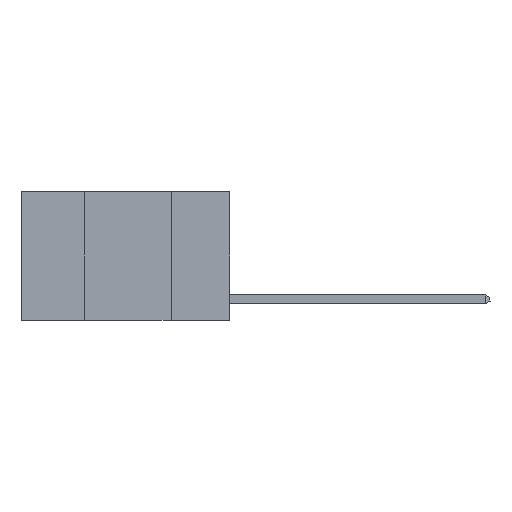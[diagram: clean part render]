
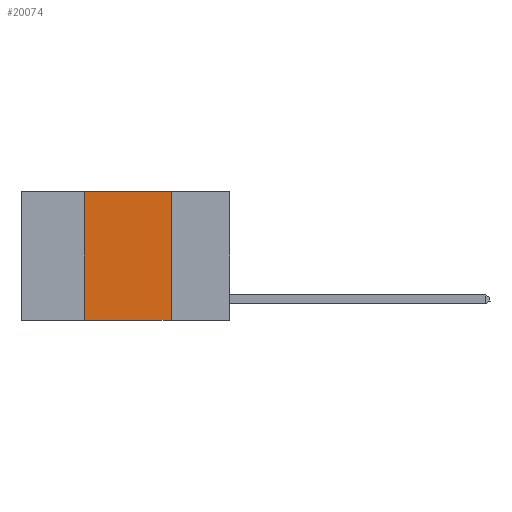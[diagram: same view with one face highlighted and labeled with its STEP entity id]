
A CAD part, left-side view. The second image highlights one B-rep face of the part: STEP entity #20074.
In plain terms, the highlighted planar face has unit normal (-1, 0, 0).
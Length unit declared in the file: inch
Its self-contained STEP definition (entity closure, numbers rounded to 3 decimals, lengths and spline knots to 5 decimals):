
#1124 = ORIENTED_EDGE ( 'NONE', *, *, #6779, .F. ) ;
#2947 = VERTEX_POINT ( 'NONE', #5891 ) ;
#3557 = ORIENTED_EDGE ( 'NONE', *, *, #16821, .T. ) ;
#3679 = VERTEX_POINT ( 'NONE', #15670 ) ;
#3696 = CARTESIAN_POINT ( 'NONE',  ( 0., 0.6, 0. ) ) ;
#5827 = VECTOR ( 'NONE', #14169, 39.37008 ) ;
#5891 = CARTESIAN_POINT ( 'NONE',  ( 0., 0.17, -0.37 ) ) ;
#6779 = EDGE_CURVE ( 'NONE', #3679, #17663, #15502, .T. ) ;
#7048 = CARTESIAN_POINT ( 'NONE',  ( 0., 0.6, 0. ) ) ;
#7406 = AXIS2_PLACEMENT_3D ( 'NONE', #7048, #8895, #21482 ) ;
#7772 = VECTOR ( 'NONE', #23227, 39.37008 ) ;
#7928 = VERTEX_POINT ( 'NONE', #10152 ) ;
#8895 = DIRECTION ( 'NONE',  ( 1., 0., 0. ) ) ;
#9037 = LINE ( 'NONE', #9591, #18083 ) ;
#9591 = CARTESIAN_POINT ( 'NONE',  ( 0., 0.17, 0. ) ) ;
#9761 = CARTESIAN_POINT ( 'NONE',  ( 0., 0.42, 0. ) ) ;
#10152 = CARTESIAN_POINT ( 'NONE',  ( 0., 0.17, 0. ) ) ;
#10244 = EDGE_CURVE ( 'NONE', #17663, #7928, #10326, .T. ) ;
#10326 = LINE ( 'NONE', #3696, #19339 ) ;
#12634 = LINE ( 'NONE', #16142, #7772 ) ;
#14169 = DIRECTION ( 'NONE',  ( 0., 0., 1. ) ) ;
#14608 = DIRECTION ( 'NONE',  ( 0., -1., 0. ) ) ;
#14782 = EDGE_CURVE ( 'NONE', #7928, #2947, #9037, .T. ) ;
#15502 = LINE ( 'NONE', #15904, #5827 ) ;
#15670 = CARTESIAN_POINT ( 'NONE',  ( 0., 0.42, -0.37 ) ) ;
#15904 = CARTESIAN_POINT ( 'NONE',  ( 0., 0.42, 0. ) ) ;
#16142 = CARTESIAN_POINT ( 'NONE',  ( 0., 0.6, -0.37 ) ) ;
#16821 = EDGE_CURVE ( 'NONE', #3679, #2947, #12634, .T. ) ;
#17663 = VERTEX_POINT ( 'NONE', #9761 ) ;
#17904 = PLANE ( 'NONE',  #7406 ) ;
#18083 = VECTOR ( 'NONE', #20388, 39.37008 ) ;
#18151 = ORIENTED_EDGE ( 'NONE', *, *, #10244, .F. ) ;
#19339 = VECTOR ( 'NONE', #14608, 39.37008 ) ;
#19424 = ORIENTED_EDGE ( 'NONE', *, *, #14782, .F. ) ;
#20074 = ADVANCED_FACE ( 'NONE', ( #21466 ), #17904, .F. ) ;
#20388 = DIRECTION ( 'NONE',  ( 0., 0., -1. ) ) ;
#21124 = EDGE_LOOP ( 'NONE', ( #19424, #18151, #1124, #3557 ) ) ;
#21466 = FACE_OUTER_BOUND ( 'NONE', #21124, .T. ) ;
#21482 = DIRECTION ( 'NONE',  ( 0., 0., -1. ) ) ;
#23227 = DIRECTION ( 'NONE',  ( 0., -1., 0. ) ) ;
